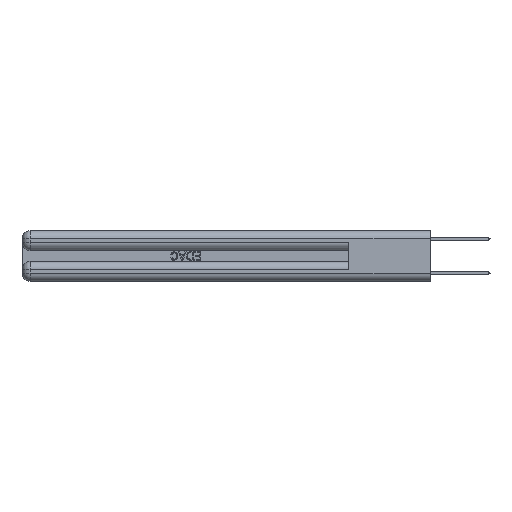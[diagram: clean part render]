
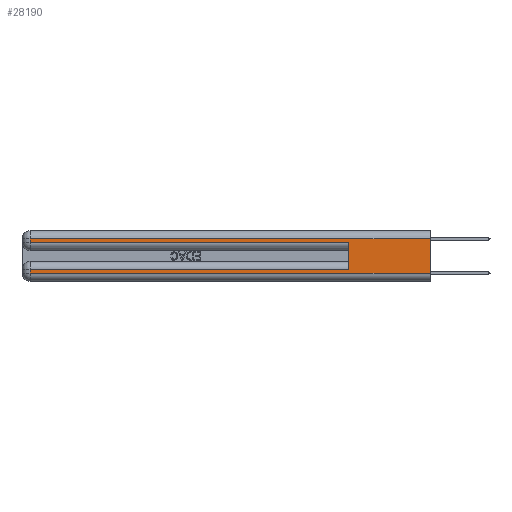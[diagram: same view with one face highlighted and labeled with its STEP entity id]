
A CAD part, left-side view. The second image highlights one B-rep face of the part: STEP entity #28190.
In plain terms, the highlighted planar face has unit normal (-1, 0, 0).
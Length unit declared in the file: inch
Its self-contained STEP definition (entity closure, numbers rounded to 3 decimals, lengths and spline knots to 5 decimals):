
#2 = ORIENTED_EDGE ( 'NONE', *, *, #27801, .T. ) ;
#125 = EDGE_CURVE ( 'NONE', #7623, #19494, #4688, .T. ) ;
#477 = CARTESIAN_POINT ( 'NONE',  ( 0., 0., 0.37 ) ) ;
#480 = CARTESIAN_POINT ( 'NONE',  ( 0., 0., 0.06 ) ) ;
#782 = VERTEX_POINT ( 'NONE', #23149 ) ;
#1120 = CARTESIAN_POINT ( 'NONE',  ( 0., 0., 0.37 ) ) ;
#1608 = LINE ( 'NONE', #2044, #10631 ) ;
#2044 = CARTESIAN_POINT ( 'NONE',  ( 0., 2.94, 0.37 ) ) ;
#2343 = DIRECTION ( 'NONE',  ( 0., 0., -1. ) ) ;
#2473 = LINE ( 'NONE', #2939, #26362 ) ;
#2562 = ORIENTED_EDGE ( 'NONE', *, *, #19603, .F. ) ;
#2939 = CARTESIAN_POINT ( 'NONE',  ( 0., 0., 0.06 ) ) ;
#3196 = VERTEX_POINT ( 'NONE', #16532 ) ;
#3527 = EDGE_CURVE ( 'NONE', #782, #30252, #1608, .T. ) ;
#4357 = VERTEX_POINT ( 'NONE', #16234 ) ;
#4580 = ORIENTED_EDGE ( 'NONE', *, *, #11471, .F. ) ;
#4688 = LINE ( 'NONE', #6908, #5662 ) ;
#5102 = EDGE_CURVE ( 'NONE', #3196, #782, #27457, .T. ) ;
#5368 = DIRECTION ( 'NONE',  ( 1., 0., 0. ) ) ;
#5631 = LINE ( 'NONE', #19483, #7394 ) ;
#5662 = VECTOR ( 'NONE', #2343, 39.37008 ) ;
#6888 = ORIENTED_EDGE ( 'NONE', *, *, #5102, .T. ) ;
#6908 = CARTESIAN_POINT ( 'NONE',  ( 0., 2.94, 0.37 ) ) ;
#7394 = VECTOR ( 'NONE', #14909, 39.37008 ) ;
#7623 = VERTEX_POINT ( 'NONE', #14247 ) ;
#7732 = DIRECTION ( 'NONE',  ( 0., 0., -1. ) ) ;
#7825 = CARTESIAN_POINT ( 'NONE',  ( 0., 0.6, 0.145 ) ) ;
#7873 = ORIENTED_EDGE ( 'NONE', *, *, #3527, .T. ) ;
#8240 = VERTEX_POINT ( 'NONE', #26862 ) ;
#8939 = CARTESIAN_POINT ( 'NONE',  ( 0., 2.94, 0.06 ) ) ;
#10631 = VECTOR ( 'NONE', #30911, 39.37008 ) ;
#11471 = EDGE_CURVE ( 'NONE', #4357, #29574, #28103, .T. ) ;
#11567 = EDGE_CURVE ( 'NONE', #30252, #29574, #2473, .T. ) ;
#11853 = VECTOR ( 'NONE', #29189, 39.37008 ) ;
#12622 = CARTESIAN_POINT ( 'NONE',  ( 0., 0., 0.285 ) ) ;
#14247 = CARTESIAN_POINT ( 'NONE',  ( 0., 2.94, 0.31 ) ) ;
#14859 = VECTOR ( 'NONE', #22972, 39.37008 ) ;
#14909 = DIRECTION ( 'NONE',  ( 0., 1., 0. ) ) ;
#14981 = DIRECTION ( 'NONE',  ( 0., -1., 0. ) ) ;
#15391 = CARTESIAN_POINT ( 'NONE',  ( 0., 0., 0.085 ) ) ;
#16119 = EDGE_LOOP ( 'NONE', ( #4580, #27912, #21729, #2, #2562, #6888, #7873, #17547 ) ) ;
#16234 = CARTESIAN_POINT ( 'NONE',  ( 0., 0., 0.31 ) ) ;
#16532 = CARTESIAN_POINT ( 'NONE',  ( 0., 0.6, 0.085 ) ) ;
#17079 = DIRECTION ( 'NONE',  ( 0., 0., 1. ) ) ;
#17547 = ORIENTED_EDGE ( 'NONE', *, *, #11567, .T. ) ;
#18496 = VECTOR ( 'NONE', #14981, 39.37008 ) ;
#19158 = DIRECTION ( 'NONE',  ( 0., -1., 0. ) ) ;
#19483 = CARTESIAN_POINT ( 'NONE',  ( 0., 0., 0.31 ) ) ;
#19494 = VERTEX_POINT ( 'NONE', #26330 ) ;
#19603 = EDGE_CURVE ( 'NONE', #3196, #8240, #24292, .T. ) ;
#19670 = PLANE ( 'NONE',  #22978 ) ;
#21284 = VECTOR ( 'NONE', #17079, 39.37008 ) ;
#21729 = ORIENTED_EDGE ( 'NONE', *, *, #125, .T. ) ;
#22972 = DIRECTION ( 'NONE',  ( 0., 0., -1. ) ) ;
#22978 = AXIS2_PLACEMENT_3D ( 'NONE', #477, #5368, #7732 ) ;
#23149 = CARTESIAN_POINT ( 'NONE',  ( 0., 2.94, 0.085 ) ) ;
#24292 = LINE ( 'NONE', #7825, #21284 ) ;
#24523 = FACE_OUTER_BOUND ( 'NONE', #16119, .T. ) ;
#26330 = CARTESIAN_POINT ( 'NONE',  ( 0., 2.94, 0.285 ) ) ;
#26362 = VECTOR ( 'NONE', #19158, 39.37008 ) ;
#26862 = CARTESIAN_POINT ( 'NONE',  ( 0., 0.6, 0.285 ) ) ;
#27051 = LINE ( 'NONE', #12622, #18496 ) ;
#27457 = LINE ( 'NONE', #15391, #11853 ) ;
#27801 = EDGE_CURVE ( 'NONE', #19494, #8240, #27051, .T. ) ;
#27912 = ORIENTED_EDGE ( 'NONE', *, *, #28745, .T. ) ;
#28103 = LINE ( 'NONE', #1120, #14859 ) ;
#28190 = ADVANCED_FACE ( 'NONE', ( #24523 ), #19670, .F. ) ;
#28745 = EDGE_CURVE ( 'NONE', #4357, #7623, #5631, .T. ) ;
#29189 = DIRECTION ( 'NONE',  ( 0., 1., 0. ) ) ;
#29574 = VERTEX_POINT ( 'NONE', #480 ) ;
#30252 = VERTEX_POINT ( 'NONE', #8939 ) ;
#30911 = DIRECTION ( 'NONE',  ( 0., 0., -1. ) ) ;
